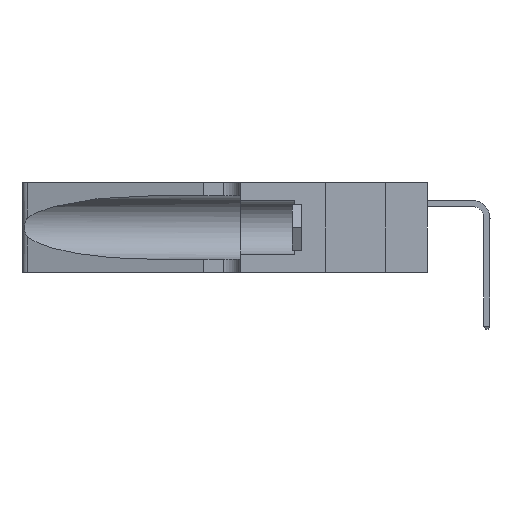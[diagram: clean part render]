
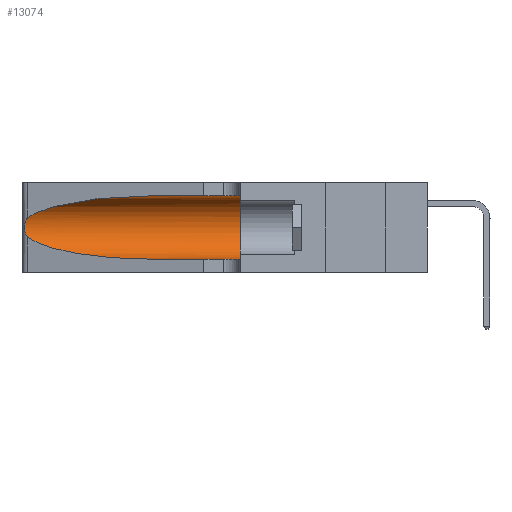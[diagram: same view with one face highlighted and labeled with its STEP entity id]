
A CAD part, left-side view. The second image highlights one B-rep face of the part: STEP entity #13074.
In plain terms, the highlighted cylindrical face has radius 3.308 mm (diameter 6.617 mm), a partial arc.
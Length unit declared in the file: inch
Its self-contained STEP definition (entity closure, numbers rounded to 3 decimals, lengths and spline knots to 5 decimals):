
#194 = EDGE_CURVE ( 'NONE', #13664, #21939, #20597, .T. ) ;
#629 = ORIENTED_EDGE ( 'NONE', *, *, #26051, .T. ) ;
#641 = B_SPLINE_CURVE_WITH_KNOTS ( 'NONE', 3,
 ( #37307, #7807, #31686, #13840, #34618, #16856, #37554, #19876, #1933, #22826, #4911, #25816, #7940, #28814 ),
 .UNSPECIFIED., .F., .F.,
 ( 4, 2, 2, 2, 2, 2, 4 ),
 ( 0., 0.00027, 0.00053, 0.00107, 0.0016, 0.00187, 0.00214 ),
 .UNSPECIFIED. ) ;
#1274 = CARTESIAN_POINT ( 'NONE',  ( 0.1305, 0.72297, 0.05475 ) ) ;
#1619 = CARTESIAN_POINT ( 'NONE',  ( 0.1305, 0.35, 0.05475 ) ) ;
#1933 = CARTESIAN_POINT ( 'NONE',  ( 0.26017, 1.23833, 0.17102 ) ) ;
#2966 = CARTESIAN_POINT ( 'NONE',  ( 0.2373, 1.15595, 0.28018 ) ) ;
#3297 = CARTESIAN_POINT ( 'NONE',  ( 0.1305, 0.35, 0.185 ) ) ;
#4911 = CARTESIAN_POINT ( 'NONE',  ( 0.25789, 1.23486, 0.15765 ) ) ;
#5259 = VERTEX_POINT ( 'NONE', #12532 ) ;
#5482 = AXIS2_PLACEMENT_3D ( 'NONE', #16085, #31052, #28050 ) ;
#6298 = DIRECTION ( 'NONE',  ( 0., 0., 1. ) ) ;
#6772 = CARTESIAN_POINT ( 'NONE',  ( 0.1305, 0.35, 0.31525 ) ) ;
#7807 = CARTESIAN_POINT ( 'NONE',  ( 0.25555, 1.22994, 0.2215 ) ) ;
#7940 = CARTESIAN_POINT ( 'NONE',  ( 0.25555, 1.22993, 0.14849 ) ) ;
#8481 = VECTOR ( 'NONE', #12038, 39.37008 ) ;
#8699 = CARTESIAN_POINT ( 'NONE',  ( 0.1305, 1.61858, 0.05475 ) ) ;
#9016 = CARTESIAN_POINT ( 'NONE',  ( 0.1305, 1.61858, 0.31525 ) ) ;
#9421 = LINE ( 'NONE', #9016, #8481 ) ;
#10100 = EDGE_CURVE ( 'NONE', #16446, #30345, #28652, .T. ) ;
#10515 = ORIENTED_EDGE ( 'NONE', *, *, #18093, .F. ) ;
#11706 = DIRECTION ( 'NONE',  ( 0., -1., 0. ) ) ;
#12024 = CARTESIAN_POINT ( 'NONE',  ( 0.1305, 0.72297, 0.05475 ) ) ;
#12038 = DIRECTION ( 'NONE',  ( 0., -1., 0. ) ) ;
#12122 = ORIENTED_EDGE ( 'NONE', *, *, #23735, .T. ) ;
#12216 = AXIS2_PLACEMENT_3D ( 'NONE', #3297, #24210, #6298 ) ;
#12532 = CARTESIAN_POINT ( 'NONE',  ( 0.25487, 1.22718, 0.14631 ) ) ;
#13074 = ADVANCED_FACE ( 'NONE', ( #28398 ), #27466, .F. ) ;
#13175 = CARTESIAN_POINT ( 'NONE',  ( 0.2373, 1.15595, 0.08982 ) ) ;
#13427 = ORIENTED_EDGE ( 'NONE', *, *, #36466, .T. ) ;
#13664 = VERTEX_POINT ( 'NONE', #30733 ) ;
#13840 = CARTESIAN_POINT ( 'NONE',  ( 0.25787, 1.23484, 0.2124 ) ) ;
#13848 = LINE ( 'NONE', #8699, #28749 ) ;
#16085 = CARTESIAN_POINT ( 'NONE',  ( 0.1305, 1.61858, 0.185 ) ) ;
#16446 = VERTEX_POINT ( 'NONE', #6772 ) ;
#16856 = CARTESIAN_POINT ( 'NONE',  ( 0.26018, 1.23835, 0.19895 ) ) ;
#17251 = ORIENTED_EDGE ( 'NONE', *, *, #194, .T. ) ;
#18093 = EDGE_CURVE ( 'NONE', #13664, #16446, #9421, .T. ) ;
#18320 =( BOUNDED_CURVE ( )  B_SPLINE_CURVE ( 3, ( #33985, #13175, #19210, #1274 ),
 .UNSPECIFIED., .F., .T. ) 
 B_SPLINE_CURVE_WITH_KNOTS ( ( 4, 4 ),
 ( 3.44316, 4.71239 ),
 .UNSPECIFIED. ) 
 CURVE ( )  GEOMETRIC_REPRESENTATION_ITEM ( )  RATIONAL_B_SPLINE_CURVE ( ( 1., 0.87, 0.87, 1. ) ) 
 REPRESENTATION_ITEM ( '' )  );
#19210 = CARTESIAN_POINT ( 'NONE',  ( 0.18966, 0.96281, 0.05475 ) ) ;
#19876 = CARTESIAN_POINT ( 'NONE',  ( 0.26075, 1.23896, 0.178 ) ) ;
#20597 =( BOUNDED_CURVE ( )  B_SPLINE_CURVE ( 3, ( #35661, #23891, #2966, #25911 ),
 .UNSPECIFIED., .F., .T. ) 
 B_SPLINE_CURVE_WITH_KNOTS ( ( 4, 4 ),
 ( 1.5708, 2.84003 ),
 .UNSPECIFIED. ) 
 CURVE ( )  GEOMETRIC_REPRESENTATION_ITEM ( )  RATIONAL_B_SPLINE_CURVE ( ( 1., 0.87, 0.87, 1. ) ) 
 REPRESENTATION_ITEM ( '' )  );
#21939 = VERTEX_POINT ( 'NONE', #26950 ) ;
#22826 = CARTESIAN_POINT ( 'NONE',  ( 0.25856, 1.23593, 0.16098 ) ) ;
#23735 = EDGE_CURVE ( 'NONE', #5259, #31333, #18320, .T. ) ;
#23891 = CARTESIAN_POINT ( 'NONE',  ( 0.18966, 0.96281, 0.31525 ) ) ;
#24210 = DIRECTION ( 'NONE',  ( 0., 1., 0. ) ) ;
#25816 = CARTESIAN_POINT ( 'NONE',  ( 0.25639, 1.23186, 0.15144 ) ) ;
#25911 = CARTESIAN_POINT ( 'NONE',  ( 0.25487, 1.22718, 0.22369 ) ) ;
#26051 = EDGE_CURVE ( 'NONE', #31333, #30345, #13848, .T. ) ;
#26950 = CARTESIAN_POINT ( 'NONE',  ( 0.25487, 1.22718, 0.22369 ) ) ;
#27466 = CYLINDRICAL_SURFACE ( 'NONE', #5482, 0.13025 ) ;
#27610 = EDGE_LOOP ( 'NONE', ( #17251, #13427, #12122, #629, #31643, #10515 ) ) ;
#28050 = DIRECTION ( 'NONE',  ( 0., 0., -1. ) ) ;
#28398 = FACE_OUTER_BOUND ( 'NONE', #27610, .T. ) ;
#28652 = CIRCLE ( 'NONE', #12216, 0.13025 ) ;
#28749 = VECTOR ( 'NONE', #11706, 39.37008 ) ;
#28814 = CARTESIAN_POINT ( 'NONE',  ( 0.25487, 1.22718, 0.14631 ) ) ;
#30345 = VERTEX_POINT ( 'NONE', #1619 ) ;
#30733 = CARTESIAN_POINT ( 'NONE',  ( 0.1305, 0.72297, 0.31525 ) ) ;
#31052 = DIRECTION ( 'NONE',  ( 0., -1., 0. ) ) ;
#31333 = VERTEX_POINT ( 'NONE', #12024 ) ;
#31643 = ORIENTED_EDGE ( 'NONE', *, *, #10100, .F. ) ;
#31686 = CARTESIAN_POINT ( 'NONE',  ( 0.25639, 1.23184, 0.21858 ) ) ;
#33985 = CARTESIAN_POINT ( 'NONE',  ( 0.25487, 1.22718, 0.14631 ) ) ;
#34618 = CARTESIAN_POINT ( 'NONE',  ( 0.25854, 1.2359, 0.20912 ) ) ;
#35661 = CARTESIAN_POINT ( 'NONE',  ( 0.1305, 0.72297, 0.31525 ) ) ;
#36466 = EDGE_CURVE ( 'NONE', #21939, #5259, #641, .T. ) ;
#37307 = CARTESIAN_POINT ( 'NONE',  ( 0.25487, 1.22718, 0.22369 ) ) ;
#37554 = CARTESIAN_POINT ( 'NONE',  ( 0.26075, 1.23896, 0.19203 ) ) ;
